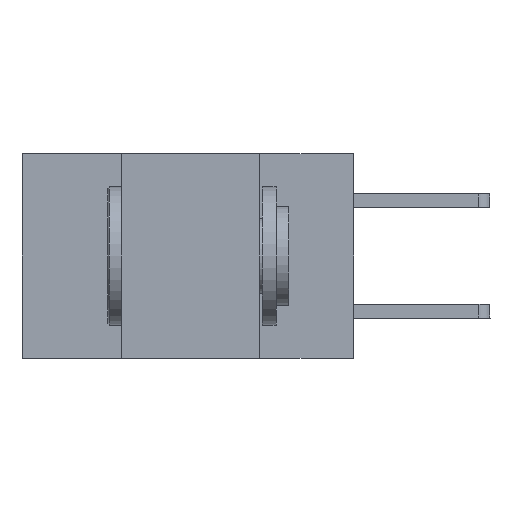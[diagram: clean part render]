
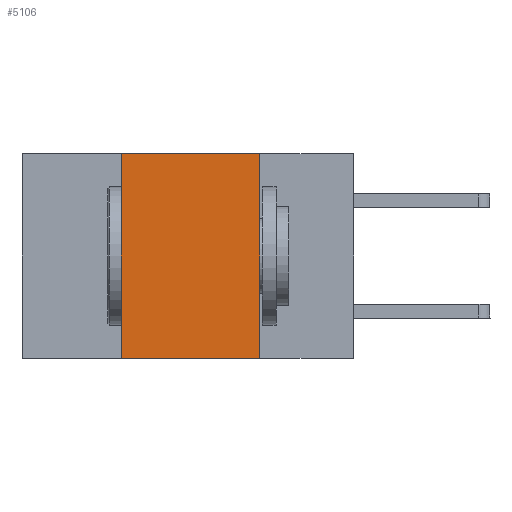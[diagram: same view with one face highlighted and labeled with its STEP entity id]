
A CAD part, left-side view. The second image highlights one B-rep face of the part: STEP entity #5106.
In plain terms, the highlighted planar face has unit normal (-1, 0, 0).
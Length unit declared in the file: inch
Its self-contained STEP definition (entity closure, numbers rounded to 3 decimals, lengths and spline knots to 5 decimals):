
#987 = VERTEX_POINT ( 'NONE', #12699 ) ;
#1066 = ORIENTED_EDGE ( 'NONE', *, *, #5953, .F. ) ;
#1344 = ORIENTED_EDGE ( 'NONE', *, *, #3501, .T. ) ;
#2328 = AXIS2_PLACEMENT_3D ( 'NONE', #9813, #10896, #2601 ) ;
#2498 = DIRECTION ( 'NONE',  ( 0., 0., 1. ) ) ;
#2601 = DIRECTION ( 'NONE',  ( 0., 0., -1. ) ) ;
#3440 = VECTOR ( 'NONE', #4610, 39.37008 ) ;
#3501 = EDGE_CURVE ( 'NONE', #6910, #7058, #8706, .T. ) ;
#3773 = ORIENTED_EDGE ( 'NONE', *, *, #13428, .F. ) ;
#4055 = CARTESIAN_POINT ( 'NONE',  ( 0., 0.17, -0.37 ) ) ;
#4358 = FACE_OUTER_BOUND ( 'NONE', #13192, .T. ) ;
#4359 = VERTEX_POINT ( 'NONE', #9115 ) ;
#4610 = DIRECTION ( 'NONE',  ( 0., -1., 0. ) ) ;
#5106 = ADVANCED_FACE ( 'NONE', ( #4358 ), #5639, .F. ) ;
#5130 = ORIENTED_EDGE ( 'NONE', *, *, #7663, .F. ) ;
#5155 = CARTESIAN_POINT ( 'NONE',  ( 0., 0.6, 0. ) ) ;
#5639 = PLANE ( 'NONE',  #2328 ) ;
#5953 = EDGE_CURVE ( 'NONE', #987, #7058, #8835, .T. ) ;
#6580 = VECTOR ( 'NONE', #9384, 39.37008 ) ;
#6892 = CARTESIAN_POINT ( 'NONE',  ( 0., 0.17, 0. ) ) ;
#6910 = VERTEX_POINT ( 'NONE', #12028 ) ;
#7058 = VERTEX_POINT ( 'NONE', #4055 ) ;
#7663 = EDGE_CURVE ( 'NONE', #4359, #987, #13261, .T. ) ;
#8111 = VECTOR ( 'NONE', #2498, 39.37008 ) ;
#8706 = LINE ( 'NONE', #12862, #3440 ) ;
#8835 = LINE ( 'NONE', #6892, #11744 ) ;
#8996 = LINE ( 'NONE', #13159, #8111 ) ;
#9115 = CARTESIAN_POINT ( 'NONE',  ( 0., 0.42, 0. ) ) ;
#9384 = DIRECTION ( 'NONE',  ( 0., -1., 0. ) ) ;
#9813 = CARTESIAN_POINT ( 'NONE',  ( 0., 0.6, 0. ) ) ;
#10896 = DIRECTION ( 'NONE',  ( 1., 0., 0. ) ) ;
#11744 = VECTOR ( 'NONE', #11960, 39.37008 ) ;
#11960 = DIRECTION ( 'NONE',  ( 0., 0., -1. ) ) ;
#12028 = CARTESIAN_POINT ( 'NONE',  ( 0., 0.42, -0.37 ) ) ;
#12699 = CARTESIAN_POINT ( 'NONE',  ( 0., 0.17, 0. ) ) ;
#12862 = CARTESIAN_POINT ( 'NONE',  ( 0., 0.6, -0.37 ) ) ;
#13159 = CARTESIAN_POINT ( 'NONE',  ( 0., 0.42, 0. ) ) ;
#13192 = EDGE_LOOP ( 'NONE', ( #1066, #5130, #3773, #1344 ) ) ;
#13261 = LINE ( 'NONE', #5155, #6580 ) ;
#13428 = EDGE_CURVE ( 'NONE', #6910, #4359, #8996, .T. ) ;
